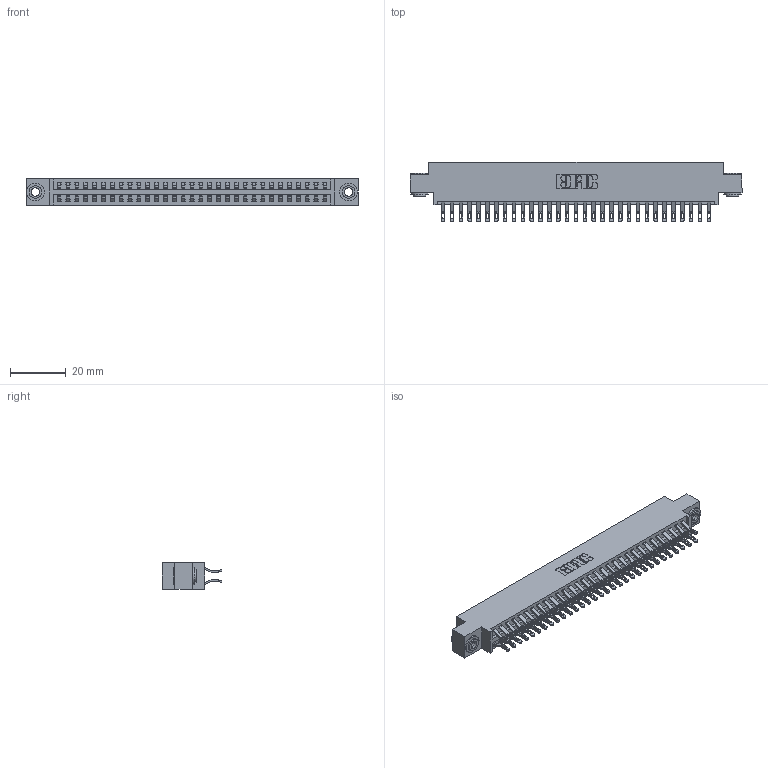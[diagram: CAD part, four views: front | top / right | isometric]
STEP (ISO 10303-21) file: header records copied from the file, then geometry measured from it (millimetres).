
FILE_DESCRIPTION (( 'STEP AP203' ), '1' );
FILE_NAME ('396-062-555-803.STEP', '2019-11-02T09:26:50', ( '' ), ( '' ), 'SwSTEP 2.0', 'SolidWorks 2016', '' );
FILE_SCHEMA (( 'CONFIG_CONTROL_DESIGN' ));
Length unit declared in the file: inch
Products named in the file (4): 345-250-002_345-250-002-102; 396-062-555-803; 346 Part_0.170 Offset - 0.156 Dia-TH; 345-292-001_555 Tail
Assembly tree (65 placements, depth 2):
  396-062-555-803
    346 Part_0.170 Offset - 0.156 Dia-TH
    345-292-001_555 Tail  x62
    345-250-002_345-250-002-102  x2
Bounding box: 119 x 21.46 x 9.4 mm (x, y, z)
Volume: 11563.1 mm3; surface area: 16756.2 mm2
Topology: 65 solids, 65 shells, 3760 faces, 11763 edges, 7838 vertices
Faces by surface type: plane 2136, cylinder 1616, cone 8
Entity records: 22820 total; most frequent: CARTESIAN_POINT 3789, ORIENTED_EDGE 3686, DIRECTION 3389, EDGE_CURVE 1843, LINE 1543, VECTOR 1543, VERTEX_POINT 1226, AXIS2_PLACEMENT_3D 923
